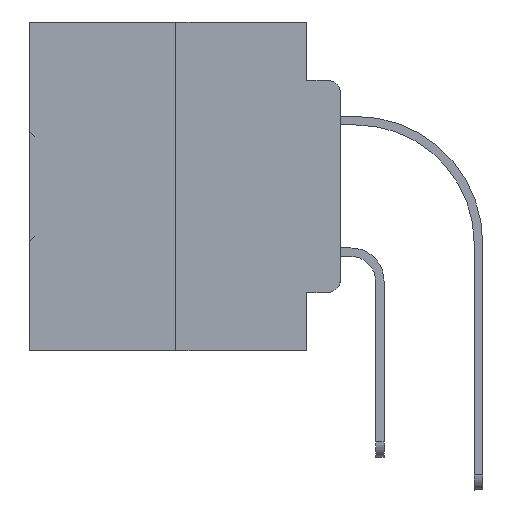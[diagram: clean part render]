
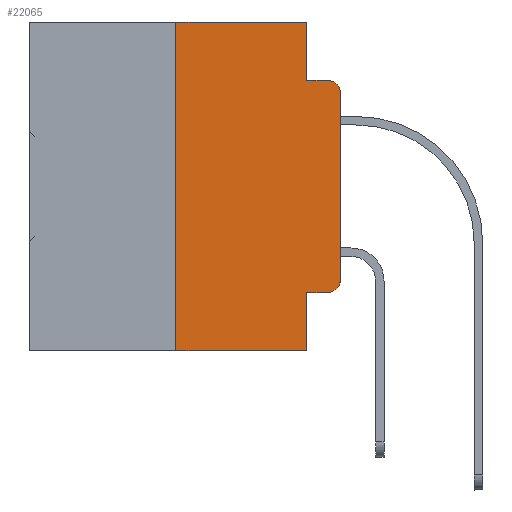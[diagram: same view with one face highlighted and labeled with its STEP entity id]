
A CAD part, left-side view. The second image highlights one B-rep face of the part: STEP entity #22065.
In plain terms, the highlighted planar face has unit normal (-1, 0, 0).
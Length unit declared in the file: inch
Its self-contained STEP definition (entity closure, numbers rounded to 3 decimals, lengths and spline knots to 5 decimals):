
#423 = EDGE_CURVE ( 'NONE', #16722, #22853, #13858, .T. ) ;
#924 = CARTESIAN_POINT ( 'NONE',  ( 0., 0.051, 0. ) ) ;
#1067 = EDGE_CURVE ( 'NONE', #27588, #5520, #21279, .T. ) ;
#1585 = AXIS2_PLACEMENT_3D ( 'NONE', #23493, #17148, #25919 ) ;
#1872 = VERTEX_POINT ( 'NONE', #5515 ) ;
#2743 = VERTEX_POINT ( 'NONE', #2784 ) ;
#2784 = CARTESIAN_POINT ( 'NONE',  ( 0., 0.25, -0.5 ) ) ;
#3747 = VERTEX_POINT ( 'NONE', #17421 ) ;
#4206 = VECTOR ( 'NONE', #25256, 39.37008 ) ;
#5448 = EDGE_CURVE ( 'NONE', #15401, #1872, #11648, .T. ) ;
#5515 = CARTESIAN_POINT ( 'NONE',  ( 0., 0.051, 0. ) ) ;
#5520 = VERTEX_POINT ( 'NONE', #9210 ) ;
#6273 = CIRCLE ( 'NONE', #1585, 0.02 ) ;
#6316 = ORIENTED_EDGE ( 'NONE', *, *, #423, .F. ) ;
#6330 = AXIS2_PLACEMENT_3D ( 'NONE', #14380, #25778, #20187 ) ;
#6376 = ORIENTED_EDGE ( 'NONE', *, *, #33652, .F. ) ;
#6763 = AXIS2_PLACEMENT_3D ( 'NONE', #33554, #35814, #10163 ) ;
#6871 = DIRECTION ( 'NONE',  ( 0., -1., 0. ) ) ;
#8074 = DIRECTION ( 'NONE',  ( 0., -1., 0. ) ) ;
#9053 = LINE ( 'NONE', #28694, #20249 ) ;
#9210 = CARTESIAN_POINT ( 'NONE',  ( 0., 0.051, -0.5 ) ) ;
#9673 = CARTESIAN_POINT ( 'NONE',  ( 0., 0., 0. ) ) ;
#9860 = LINE ( 'NONE', #14748, #20547 ) ;
#10149 = CARTESIAN_POINT ( 'NONE',  ( 0., 0.25, 0. ) ) ;
#10163 = DIRECTION ( 'NONE',  ( 0., 0., -1. ) ) ;
#10697 = VERTEX_POINT ( 'NONE', #19744 ) ;
#11648 = LINE ( 'NONE', #27560, #20026 ) ;
#12310 = CIRCLE ( 'NONE', #6330, 0.02 ) ;
#12491 = DIRECTION ( 'NONE',  ( 0., -1., 0. ) ) ;
#13147 = PLANE ( 'NONE',  #6763 ) ;
#13363 = DIRECTION ( 'NONE',  ( 0., -1., 0. ) ) ;
#13858 = LINE ( 'NONE', #22276, #32789 ) ;
#14380 = CARTESIAN_POINT ( 'NONE',  ( 0., 0.02, -0.3915 ) ) ;
#14748 = CARTESIAN_POINT ( 'NONE',  ( 0., 0.051, -0.4115 ) ) ;
#14772 = ORIENTED_EDGE ( 'NONE', *, *, #26557, .T. ) ;
#15401 = VERTEX_POINT ( 'NONE', #10149 ) ;
#15529 = ORIENTED_EDGE ( 'NONE', *, *, #5448, .F. ) ;
#16722 = VERTEX_POINT ( 'NONE', #20613 ) ;
#16885 = VECTOR ( 'NONE', #6871, 39.37008 ) ;
#17019 = ORIENTED_EDGE ( 'NONE', *, *, #24631, .T. ) ;
#17148 = DIRECTION ( 'NONE',  ( -1., 0., 0. ) ) ;
#17421 = CARTESIAN_POINT ( 'NONE',  ( 0., 0., -0.3915 ) ) ;
#17727 = LINE ( 'NONE', #29147, #16885 ) ;
#17808 = VECTOR ( 'NONE', #18292, 39.37008 ) ;
#17912 = LINE ( 'NONE', #9673, #24695 ) ;
#18292 = DIRECTION ( 'NONE',  ( 0., 0., -1. ) ) ;
#18340 = CARTESIAN_POINT ( 'NONE',  ( 0., 0.051, -0.4115 ) ) ;
#19744 = CARTESIAN_POINT ( 'NONE',  ( 0., 0.02, -0.4115 ) ) ;
#19902 = DIRECTION ( 'NONE',  ( 0., 0., 1. ) ) ;
#20026 = VECTOR ( 'NONE', #13363, 39.37008 ) ;
#20187 = DIRECTION ( 'NONE',  ( 0., 0., -1. ) ) ;
#20195 = ORIENTED_EDGE ( 'NONE', *, *, #1067, .F. ) ;
#20249 = VECTOR ( 'NONE', #19902, 39.37008 ) ;
#20547 = VECTOR ( 'NONE', #12491, 39.37008 ) ;
#20613 = CARTESIAN_POINT ( 'NONE',  ( 0., 0.051, -0.0885 ) ) ;
#21279 = LINE ( 'NONE', #924, #17808 ) ;
#22065 = ADVANCED_FACE ( 'NONE', ( #36540 ), #13147, .F. ) ;
#22276 = CARTESIAN_POINT ( 'NONE',  ( 0., 0.051, -0.0885 ) ) ;
#22853 = VERTEX_POINT ( 'NONE', #29194 ) ;
#23294 = EDGE_CURVE ( 'NONE', #2743, #5520, #17727, .T. ) ;
#23493 = CARTESIAN_POINT ( 'NONE',  ( 0., 0.02, -0.1085 ) ) ;
#24613 = EDGE_CURVE ( 'NONE', #27588, #10697, #9860, .T. ) ;
#24631 = EDGE_CURVE ( 'NONE', #3747, #35384, #17912, .T. ) ;
#24695 = VECTOR ( 'NONE', #32514, 39.37008 ) ;
#24891 = LINE ( 'NONE', #34089, #4206 ) ;
#25231 = EDGE_LOOP ( 'NONE', ( #17019, #28079, #6316, #6376, #15529, #31548, #30690, #20195, #32925, #14772 ) ) ;
#25256 = DIRECTION ( 'NONE',  ( 0., 0., -1. ) ) ;
#25778 = DIRECTION ( 'NONE',  ( -1., 0., 0. ) ) ;
#25919 = DIRECTION ( 'NONE',  ( 0., 0., -1. ) ) ;
#26557 = EDGE_CURVE ( 'NONE', #10697, #3747, #12310, .T. ) ;
#26882 = EDGE_CURVE ( 'NONE', #35384, #22853, #6273, .T. ) ;
#27560 = CARTESIAN_POINT ( 'NONE',  ( 0., 0.473, 0. ) ) ;
#27588 = VERTEX_POINT ( 'NONE', #18340 ) ;
#28079 = ORIENTED_EDGE ( 'NONE', *, *, #26882, .T. ) ;
#28694 = CARTESIAN_POINT ( 'NONE',  ( 0., 0.25, 0. ) ) ;
#29147 = CARTESIAN_POINT ( 'NONE',  ( 0., 0.473, -0.5 ) ) ;
#29194 = CARTESIAN_POINT ( 'NONE',  ( 0., 0.02, -0.0885 ) ) ;
#30690 = ORIENTED_EDGE ( 'NONE', *, *, #23294, .T. ) ;
#31548 = ORIENTED_EDGE ( 'NONE', *, *, #32321, .F. ) ;
#32321 = EDGE_CURVE ( 'NONE', #2743, #15401, #9053, .T. ) ;
#32514 = DIRECTION ( 'NONE',  ( 0., 0., 1. ) ) ;
#32789 = VECTOR ( 'NONE', #8074, 39.37008 ) ;
#32925 = ORIENTED_EDGE ( 'NONE', *, *, #24613, .T. ) ;
#33554 = CARTESIAN_POINT ( 'NONE',  ( 0., 0.473, 0. ) ) ;
#33652 = EDGE_CURVE ( 'NONE', #1872, #16722, #24891, .T. ) ;
#34089 = CARTESIAN_POINT ( 'NONE',  ( 0., 0.051, 0. ) ) ;
#35384 = VERTEX_POINT ( 'NONE', #35614 ) ;
#35614 = CARTESIAN_POINT ( 'NONE',  ( 0., 0., -0.1085 ) ) ;
#35814 = DIRECTION ( 'NONE',  ( 1., 0., 0. ) ) ;
#36540 = FACE_OUTER_BOUND ( 'NONE', #25231, .T. ) ;
